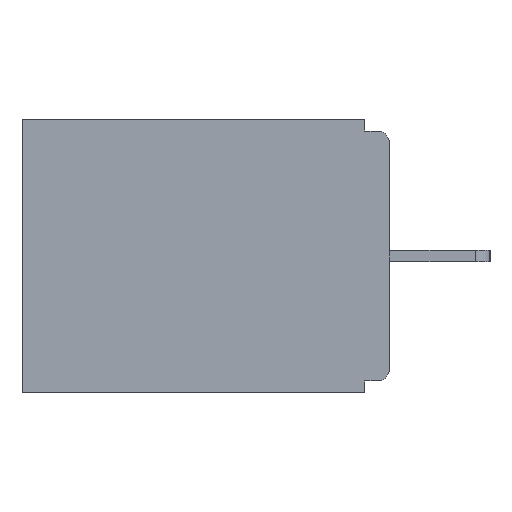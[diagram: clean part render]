
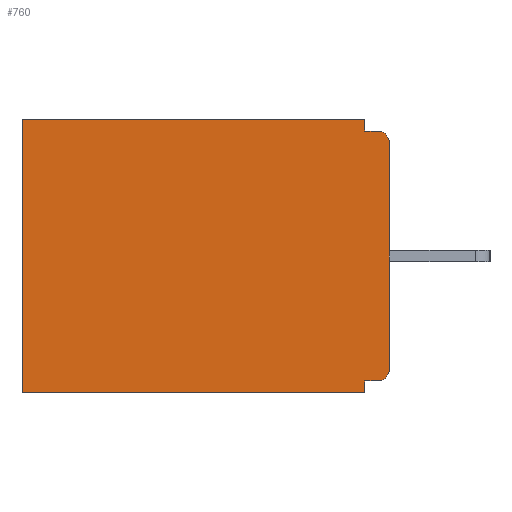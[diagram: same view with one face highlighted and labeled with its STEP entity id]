
A CAD part, left-side view. The second image highlights one B-rep face of the part: STEP entity #760.
In plain terms, the highlighted planar face has unit normal (-1, 0, 0).
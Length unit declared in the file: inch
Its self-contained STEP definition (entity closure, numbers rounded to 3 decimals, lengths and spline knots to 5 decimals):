
#19 = VECTOR ( 'NONE', #21292, 39.37008 ) ;
#74 = FACE_OUTER_BOUND ( 'NONE', #8299, .T. ) ;
#380 = CARTESIAN_POINT ( 'NONE',  ( 0.298, 0.46, -0.343 ) ) ;
#456 = VERTEX_POINT ( 'NONE', #7122 ) ;
#760 = ADVANCED_FACE ( 'NONE', ( #74 ), #8341, .F. ) ;
#1221 = VECTOR ( 'NONE', #9956, 39.37008 ) ;
#1265 = LINE ( 'NONE', #15550, #15412 ) ;
#1915 = CARTESIAN_POINT ( 'NONE',  ( 0.298, 0., -0.328 ) ) ;
#1931 = LINE ( 'NONE', #22215, #11165 ) ;
#2202 = ORIENTED_EDGE ( 'NONE', *, *, #12882, .F. ) ;
#2262 = ORIENTED_EDGE ( 'NONE', *, *, #4223, .F. ) ;
#2319 = ORIENTED_EDGE ( 'NONE', *, *, #4638, .F. ) ;
#2618 = VERTEX_POINT ( 'NONE', #380 ) ;
#2784 = CARTESIAN_POINT ( 'NONE',  ( 0.298, 0.031, -0.328 ) ) ;
#4223 = EDGE_CURVE ( 'NONE', #17614, #4658, #14952, .T. ) ;
#4541 = AXIS2_PLACEMENT_3D ( 'NONE', #19233, #15927, #15780 ) ;
#4638 = EDGE_CURVE ( 'NONE', #4658, #2618, #1931, .T. ) ;
#4658 = VERTEX_POINT ( 'NONE', #19458 ) ;
#4760 = VECTOR ( 'NONE', #14338, 39.37008 ) ;
#4930 = CARTESIAN_POINT ( 'NONE',  ( 0.298, 0., 0. ) ) ;
#5208 = EDGE_CURVE ( 'NONE', #456, #7564, #12639, .T. ) ;
#5343 = LINE ( 'NONE', #12503, #4760 ) ;
#6781 = CARTESIAN_POINT ( 'NONE',  ( 0.298, 0., -0.313 ) ) ;
#6846 = CARTESIAN_POINT ( 'NONE',  ( 0.298, 0.031, 0. ) ) ;
#7122 = CARTESIAN_POINT ( 'NONE',  ( 0.298, 0.015, -0.328 ) ) ;
#7318 = DIRECTION ( 'NONE',  ( 1., 0., 0. ) ) ;
#7563 = DIRECTION ( 'NONE',  ( 0., 0., -1. ) ) ;
#7564 = VERTEX_POINT ( 'NONE', #6781 ) ;
#7640 = DIRECTION ( 'NONE',  ( 0., 0., -1. ) ) ;
#7677 = VECTOR ( 'NONE', #18016, 39.37008 ) ;
#7777 = CARTESIAN_POINT ( 'NONE',  ( 0.298, 0.031, -0.343 ) ) ;
#8299 = EDGE_LOOP ( 'NONE', ( #23557, #12824, #21559, #22030, #8592, #2319, #2262, #18044, #22284, #2202 ) ) ;
#8341 = PLANE ( 'NONE',  #8617 ) ;
#8592 = ORIENTED_EDGE ( 'NONE', *, *, #17763, .T. ) ;
#8617 = AXIS2_PLACEMENT_3D ( 'NONE', #11126, #7318, #7563 ) ;
#9110 = DIRECTION ( 'NONE',  ( -1., 0., 0. ) ) ;
#9197 = VECTOR ( 'NONE', #12952, 39.37008 ) ;
#9289 = CARTESIAN_POINT ( 'NONE',  ( 0.298, 0.015, -0.313 ) ) ;
#9651 = EDGE_CURVE ( 'NONE', #14756, #14728, #9700, .T. ) ;
#9700 = CIRCLE ( 'NONE', #4541, 0.015 ) ;
#9803 = EDGE_CURVE ( 'NONE', #10422, #14728, #1265, .T. ) ;
#9956 = DIRECTION ( 'NONE',  ( 0., 0., -1. ) ) ;
#10067 = VECTOR ( 'NONE', #18222, 39.37008 ) ;
#10422 = VERTEX_POINT ( 'NONE', #13087 ) ;
#11126 = CARTESIAN_POINT ( 'NONE',  ( 0.298, 0., 0. ) ) ;
#11165 = VECTOR ( 'NONE', #22602, 39.37008 ) ;
#12503 = CARTESIAN_POINT ( 'NONE',  ( 0.298, 0.46, 0. ) ) ;
#12603 = CARTESIAN_POINT ( 'NONE',  ( 0.298, 0.031, -0.343 ) ) ;
#12616 = LINE ( 'NONE', #12603, #7677 ) ;
#12639 = CIRCLE ( 'NONE', #16776, 0.015 ) ;
#12824 = ORIENTED_EDGE ( 'NONE', *, *, #9803, .F. ) ;
#12882 = EDGE_CURVE ( 'NONE', #14756, #7564, #20099, .T. ) ;
#12952 = DIRECTION ( 'NONE',  ( 0., 1., 0. ) ) ;
#13087 = CARTESIAN_POINT ( 'NONE',  ( 0.298, 0.031, -0.015 ) ) ;
#13179 = CARTESIAN_POINT ( 'NONE',  ( 0.298, 0., -0.03 ) ) ;
#14338 = DIRECTION ( 'NONE',  ( 0., 0., -1. ) ) ;
#14728 = VERTEX_POINT ( 'NONE', #14830 ) ;
#14756 = VERTEX_POINT ( 'NONE', #13179 ) ;
#14830 = CARTESIAN_POINT ( 'NONE',  ( 0.298, 0.015, -0.015 ) ) ;
#14952 = LINE ( 'NONE', #7777, #10067 ) ;
#15412 = VECTOR ( 'NONE', #16544, 39.37008 ) ;
#15550 = CARTESIAN_POINT ( 'NONE',  ( 0.298, 0., -0.015 ) ) ;
#15780 = DIRECTION ( 'NONE',  ( 0., 0., -1. ) ) ;
#15927 = DIRECTION ( 'NONE',  ( -1., 0., 0. ) ) ;
#16307 = CARTESIAN_POINT ( 'NONE',  ( 0.298, 0.46, 0. ) ) ;
#16506 = EDGE_CURVE ( 'NONE', #456, #17614, #18291, .T. ) ;
#16544 = DIRECTION ( 'NONE',  ( 0., -1., 0. ) ) ;
#16776 = AXIS2_PLACEMENT_3D ( 'NONE', #9289, #9110, #7640 ) ;
#17614 = VERTEX_POINT ( 'NONE', #2784 ) ;
#17763 = EDGE_CURVE ( 'NONE', #19128, #2618, #5343, .T. ) ;
#18016 = DIRECTION ( 'NONE',  ( 0., 0., -1. ) ) ;
#18044 = ORIENTED_EDGE ( 'NONE', *, *, #16506, .F. ) ;
#18222 = DIRECTION ( 'NONE',  ( 0., 0., -1. ) ) ;
#18291 = LINE ( 'NONE', #1915, #9197 ) ;
#18984 = CARTESIAN_POINT ( 'NONE',  ( 0.298, 0., 0. ) ) ;
#19128 = VERTEX_POINT ( 'NONE', #16307 ) ;
#19233 = CARTESIAN_POINT ( 'NONE',  ( 0.298, 0.015, -0.03 ) ) ;
#19458 = CARTESIAN_POINT ( 'NONE',  ( 0.298, 0.031, -0.343 ) ) ;
#19883 = EDGE_CURVE ( 'NONE', #23498, #10422, #12616, .T. ) ;
#20099 = LINE ( 'NONE', #18984, #1221 ) ;
#21292 = DIRECTION ( 'NONE',  ( 0., 1., 0. ) ) ;
#21559 = ORIENTED_EDGE ( 'NONE', *, *, #19883, .F. ) ;
#21724 = LINE ( 'NONE', #4930, #19 ) ;
#22030 = ORIENTED_EDGE ( 'NONE', *, *, #22130, .T. ) ;
#22130 = EDGE_CURVE ( 'NONE', #23498, #19128, #21724, .T. ) ;
#22215 = CARTESIAN_POINT ( 'NONE',  ( 0.298, 0., -0.343 ) ) ;
#22284 = ORIENTED_EDGE ( 'NONE', *, *, #5208, .T. ) ;
#22602 = DIRECTION ( 'NONE',  ( 0., 1., 0. ) ) ;
#23498 = VERTEX_POINT ( 'NONE', #6846 ) ;
#23557 = ORIENTED_EDGE ( 'NONE', *, *, #9651, .T. ) ;
